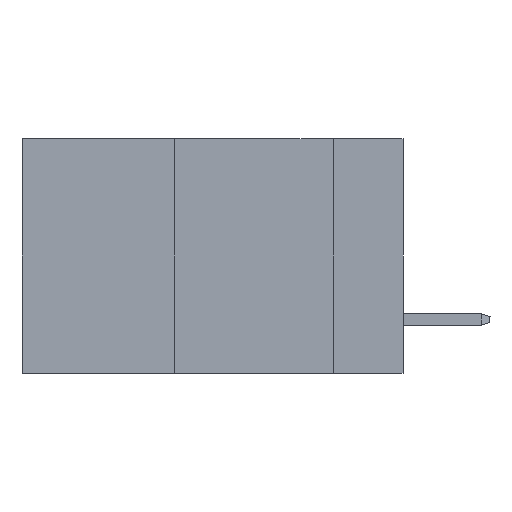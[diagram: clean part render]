
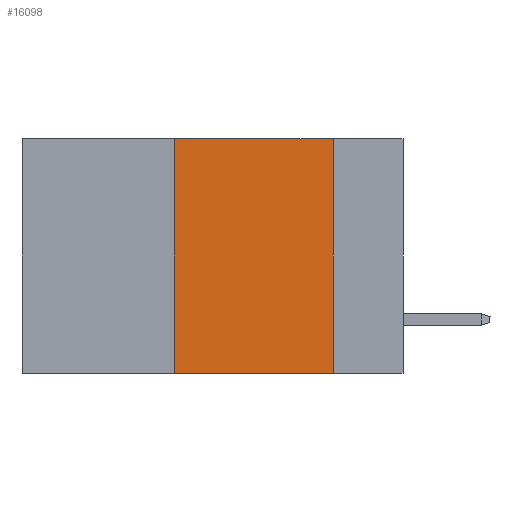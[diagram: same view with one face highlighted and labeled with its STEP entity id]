
A CAD part, left-side view. The second image highlights one B-rep face of the part: STEP entity #16098.
In plain terms, the highlighted planar face has unit normal (-1, 0, 0).
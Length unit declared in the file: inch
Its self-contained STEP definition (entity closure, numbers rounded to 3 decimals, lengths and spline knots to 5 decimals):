
#20 = ORIENTED_EDGE ( 'NONE', *, *, #3621, .F. ) ;
#389 = CARTESIAN_POINT ( 'NONE',  ( 0., 0.36, 0. ) ) ;
#784 = VECTOR ( 'NONE', #10289, 39.37008 ) ;
#1214 = CARTESIAN_POINT ( 'NONE',  ( 0., 0.11, 0. ) ) ;
#2516 = EDGE_CURVE ( 'NONE', #9084, #4460, #14225, .T. ) ;
#2795 = ORIENTED_EDGE ( 'NONE', *, *, #19902, .F. ) ;
#3281 = ORIENTED_EDGE ( 'NONE', *, *, #24932, .F. ) ;
#3621 = EDGE_CURVE ( 'NONE', #25041, #4460, #23926, .T. ) ;
#3803 = CARTESIAN_POINT ( 'NONE',  ( 0., 0.36, 0. ) ) ;
#4235 = FACE_OUTER_BOUND ( 'NONE', #7690, .T. ) ;
#4460 = VERTEX_POINT ( 'NONE', #21321 ) ;
#4526 = DIRECTION ( 'NONE',  ( 0., 0., -1. ) ) ;
#4673 = DIRECTION ( 'NONE',  ( 1., 0., 0. ) ) ;
#5163 = CARTESIAN_POINT ( 'NONE',  ( 0., 0.36, -0.37 ) ) ;
#5225 = VECTOR ( 'NONE', #13126, 39.37008 ) ;
#6629 = PLANE ( 'NONE',  #22157 ) ;
#7690 = EDGE_LOOP ( 'NONE', ( #20, #2795, #3281, #14980 ) ) ;
#8582 = CARTESIAN_POINT ( 'NONE',  ( 0., 0.6, 0. ) ) ;
#9084 = VERTEX_POINT ( 'NONE', #5163 ) ;
#10289 = DIRECTION ( 'NONE',  ( 0., 0., -1. ) ) ;
#13126 = DIRECTION ( 'NONE',  ( 0., -1., 0. ) ) ;
#13254 = CARTESIAN_POINT ( 'NONE',  ( 0., 0.6, 0. ) ) ;
#13271 = LINE ( 'NONE', #8582, #5225 ) ;
#13303 = VERTEX_POINT ( 'NONE', #3803 ) ;
#13887 = CARTESIAN_POINT ( 'NONE',  ( 0., 0.11, 0. ) ) ;
#14180 = LINE ( 'NONE', #389, #15300 ) ;
#14225 = LINE ( 'NONE', #14369, #24855 ) ;
#14369 = CARTESIAN_POINT ( 'NONE',  ( 0., 0.6, -0.37 ) ) ;
#14472 = DIRECTION ( 'NONE',  ( 0., 0., 1. ) ) ;
#14980 = ORIENTED_EDGE ( 'NONE', *, *, #2516, .T. ) ;
#15300 = VECTOR ( 'NONE', #14472, 39.37008 ) ;
#16098 = ADVANCED_FACE ( 'NONE', ( #4235 ), #6629, .F. ) ;
#18224 = DIRECTION ( 'NONE',  ( 0., -1., 0. ) ) ;
#19902 = EDGE_CURVE ( 'NONE', #13303, #25041, #13271, .T. ) ;
#21321 = CARTESIAN_POINT ( 'NONE',  ( 0., 0.11, -0.37 ) ) ;
#22157 = AXIS2_PLACEMENT_3D ( 'NONE', #13254, #4673, #4526 ) ;
#23926 = LINE ( 'NONE', #1214, #784 ) ;
#24855 = VECTOR ( 'NONE', #18224, 39.37008 ) ;
#24932 = EDGE_CURVE ( 'NONE', #9084, #13303, #14180, .T. ) ;
#25041 = VERTEX_POINT ( 'NONE', #13887 ) ;
